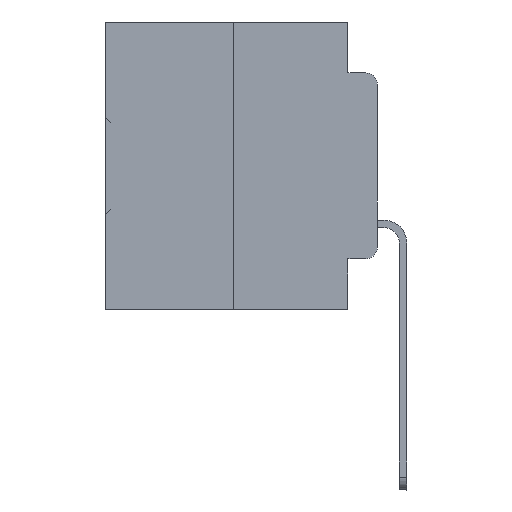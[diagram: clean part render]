
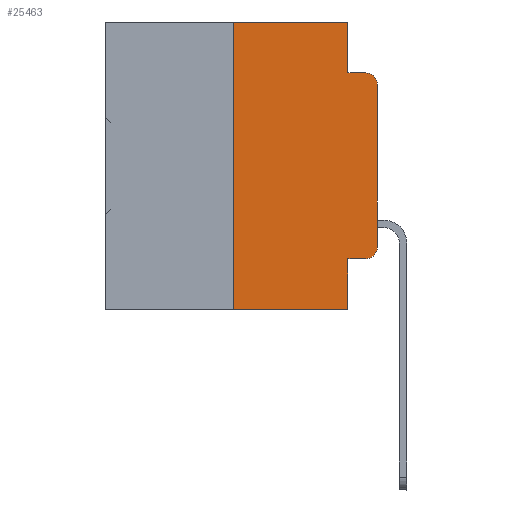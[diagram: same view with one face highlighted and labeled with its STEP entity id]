
A CAD part, left-side view. The second image highlights one B-rep face of the part: STEP entity #25463.
In plain terms, the highlighted planar face has unit normal (-1, 0, 0).
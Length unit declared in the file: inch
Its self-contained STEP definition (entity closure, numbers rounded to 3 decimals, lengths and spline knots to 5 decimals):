
#240 = EDGE_CURVE ( 'NONE', #35412, #35841, #28854, .T. ) ;
#577 = ORIENTED_EDGE ( 'NONE', *, *, #13353, .F. ) ;
#1370 = ORIENTED_EDGE ( 'NONE', *, *, #21396, .F. ) ;
#2482 = VECTOR ( 'NONE', #26535, 39.37008 ) ;
#3601 = DIRECTION ( 'NONE',  ( 0., -1., 0. ) ) ;
#4630 = VERTEX_POINT ( 'NONE', #15297 ) ;
#5324 = CARTESIAN_POINT ( 'NONE',  ( 0., 0., -0.1085 ) ) ;
#5403 = DIRECTION ( 'NONE',  ( 0., 0., -1. ) ) ;
#5628 = AXIS2_PLACEMENT_3D ( 'NONE', #22943, #16990, #16617 ) ;
#5659 = DIRECTION ( 'NONE',  ( 0., -1., 0. ) ) ;
#6446 = VERTEX_POINT ( 'NONE', #10028 ) ;
#7063 = DIRECTION ( 'NONE',  ( 0., -1., 0. ) ) ;
#7570 = EDGE_CURVE ( 'NONE', #4630, #35841, #34864, .T. ) ;
#7769 = ORIENTED_EDGE ( 'NONE', *, *, #26326, .T. ) ;
#7952 = LINE ( 'NONE', #33679, #32918 ) ;
#9019 = VERTEX_POINT ( 'NONE', #22737 ) ;
#9653 = VECTOR ( 'NONE', #16616, 39.37008 ) ;
#9727 = PLANE ( 'NONE',  #16193 ) ;
#10028 = CARTESIAN_POINT ( 'NONE',  ( 0., 0.02, -0.4115 ) ) ;
#10119 = ORIENTED_EDGE ( 'NONE', *, *, #34591, .T. ) ;
#10474 = ORIENTED_EDGE ( 'NONE', *, *, #32811, .T. ) ;
#10699 = LINE ( 'NONE', #33647, #27580 ) ;
#11149 = ORIENTED_EDGE ( 'NONE', *, *, #240, .T. ) ;
#12620 = DIRECTION ( 'NONE',  ( -1., 0., 0. ) ) ;
#12735 = VERTEX_POINT ( 'NONE', #19890 ) ;
#13353 = EDGE_CURVE ( 'NONE', #19112, #4630, #36808, .T. ) ;
#13722 = DIRECTION ( 'NONE',  ( 0., -1., 0. ) ) ;
#14594 = EDGE_CURVE ( 'NONE', #9019, #19112, #20216, .T. ) ;
#14648 = EDGE_LOOP ( 'NONE', ( #35010, #11149, #15923, #577, #15855, #1370, #10119, #19333, #10474, #7769 ) ) ;
#15178 = CARTESIAN_POINT ( 'NONE',  ( 0., 0.25, 0. ) ) ;
#15297 = CARTESIAN_POINT ( 'NONE',  ( 0., 0.051, -0.0885 ) ) ;
#15507 = DIRECTION ( 'NONE',  ( 1., 0., 0. ) ) ;
#15855 = ORIENTED_EDGE ( 'NONE', *, *, #14594, .F. ) ;
#15923 = ORIENTED_EDGE ( 'NONE', *, *, #7570, .F. ) ;
#16193 = AXIS2_PLACEMENT_3D ( 'NONE', #18672, #15507, #18484 ) ;
#16444 = VECTOR ( 'NONE', #7063, 39.37008 ) ;
#16616 = DIRECTION ( 'NONE',  ( 0., 0., 1. ) ) ;
#16617 = DIRECTION ( 'NONE',  ( 0., 0., -1. ) ) ;
#16990 = DIRECTION ( 'NONE',  ( -1., 0., 0. ) ) ;
#17172 = CARTESIAN_POINT ( 'NONE',  ( 0., 0.02, -0.0885 ) ) ;
#17361 = CARTESIAN_POINT ( 'NONE',  ( 0., 0., 0. ) ) ;
#17795 = VECTOR ( 'NONE', #19848, 39.37008 ) ;
#18377 = VECTOR ( 'NONE', #3601, 39.37008 ) ;
#18484 = DIRECTION ( 'NONE',  ( 0., 0., -1. ) ) ;
#18570 = VECTOR ( 'NONE', #5403, 39.37008 ) ;
#18672 = CARTESIAN_POINT ( 'NONE',  ( 0., 0.473, 0. ) ) ;
#19112 = VERTEX_POINT ( 'NONE', #28234 ) ;
#19333 = ORIENTED_EDGE ( 'NONE', *, *, #31911, .F. ) ;
#19848 = DIRECTION ( 'NONE',  ( 0., 0., -1. ) ) ;
#19890 = CARTESIAN_POINT ( 'NONE',  ( 0., 0.051, -0.5 ) ) ;
#20139 = CARTESIAN_POINT ( 'NONE',  ( 0., 0.051, 0. ) ) ;
#20216 = LINE ( 'NONE', #29169, #18377 ) ;
#20421 = LINE ( 'NONE', #17361, #9653 ) ;
#20460 = CARTESIAN_POINT ( 'NONE',  ( 0., 0.02, -0.3915 ) ) ;
#21227 = CARTESIAN_POINT ( 'NONE',  ( 0., 0.25, -0.5 ) ) ;
#21396 = EDGE_CURVE ( 'NONE', #30650, #9019, #35121, .T. ) ;
#22190 = AXIS2_PLACEMENT_3D ( 'NONE', #20460, #12620, #32397 ) ;
#22737 = CARTESIAN_POINT ( 'NONE',  ( 0., 0.25, 0. ) ) ;
#22943 = CARTESIAN_POINT ( 'NONE',  ( 0., 0.02, -0.1085 ) ) ;
#25463 = ADVANCED_FACE ( 'NONE', ( #32296 ), #9727, .F. ) ;
#26326 = EDGE_CURVE ( 'NONE', #6446, #27543, #31747, .T. ) ;
#26462 = CARTESIAN_POINT ( 'NONE',  ( 0., 0.051, -0.0885 ) ) ;
#26535 = DIRECTION ( 'NONE',  ( 0., 0., 1. ) ) ;
#26597 = CARTESIAN_POINT ( 'NONE',  ( 0., 0., -0.3915 ) ) ;
#27543 = VERTEX_POINT ( 'NONE', #26597 ) ;
#27580 = VECTOR ( 'NONE', #5659, 39.37008 ) ;
#28234 = CARTESIAN_POINT ( 'NONE',  ( 0., 0.051, 0. ) ) ;
#28854 = CIRCLE ( 'NONE', #5628, 0.02 ) ;
#29169 = CARTESIAN_POINT ( 'NONE',  ( 0., 0.473, 0. ) ) ;
#30650 = VERTEX_POINT ( 'NONE', #21227 ) ;
#30963 = LINE ( 'NONE', #20139, #18570 ) ;
#31527 = VERTEX_POINT ( 'NONE', #31609 ) ;
#31578 = EDGE_CURVE ( 'NONE', #27543, #35412, #20421, .T. ) ;
#31609 = CARTESIAN_POINT ( 'NONE',  ( 0., 0.051, -0.4115 ) ) ;
#31747 = CIRCLE ( 'NONE', #22190, 0.02 ) ;
#31911 = EDGE_CURVE ( 'NONE', #31527, #12735, #30963, .T. ) ;
#32296 = FACE_OUTER_BOUND ( 'NONE', #14648, .T. ) ;
#32397 = DIRECTION ( 'NONE',  ( 0., 0., -1. ) ) ;
#32811 = EDGE_CURVE ( 'NONE', #31527, #6446, #7952, .T. ) ;
#32918 = VECTOR ( 'NONE', #13722, 39.37008 ) ;
#33647 = CARTESIAN_POINT ( 'NONE',  ( 0., 0.473, -0.5 ) ) ;
#33679 = CARTESIAN_POINT ( 'NONE',  ( 0., 0.051, -0.4115 ) ) ;
#34591 = EDGE_CURVE ( 'NONE', #30650, #12735, #10699, .T. ) ;
#34864 = LINE ( 'NONE', #26462, #16444 ) ;
#35010 = ORIENTED_EDGE ( 'NONE', *, *, #31578, .T. ) ;
#35121 = LINE ( 'NONE', #15178, #2482 ) ;
#35264 = CARTESIAN_POINT ( 'NONE',  ( 0., 0.051, 0. ) ) ;
#35412 = VERTEX_POINT ( 'NONE', #5324 ) ;
#35841 = VERTEX_POINT ( 'NONE', #17172 ) ;
#36808 = LINE ( 'NONE', #35264, #17795 ) ;
